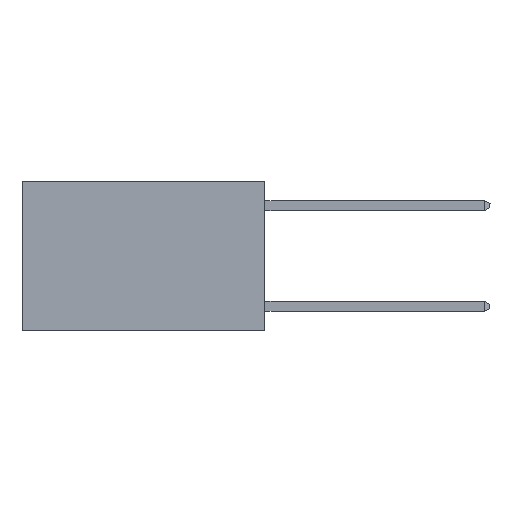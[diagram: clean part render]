
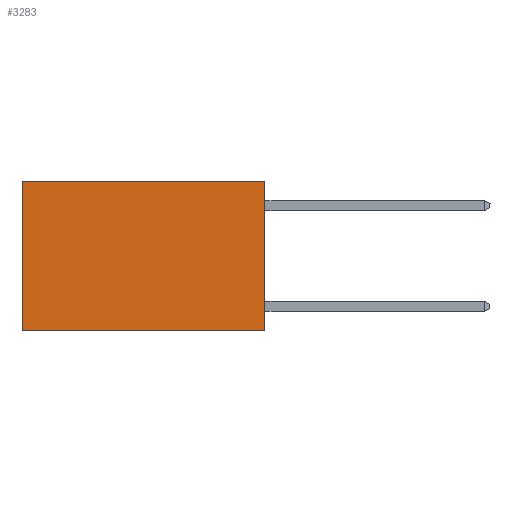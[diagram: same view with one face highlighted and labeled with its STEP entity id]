
A CAD part, left-side view. The second image highlights one B-rep face of the part: STEP entity #3283.
In plain terms, the highlighted planar face has unit normal (-1, 0, 0).
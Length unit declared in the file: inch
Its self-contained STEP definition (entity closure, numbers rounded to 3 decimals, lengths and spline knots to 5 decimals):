
#194 = VECTOR ( 'NONE', #4864, 39.37008 ) ;
#384 = CARTESIAN_POINT ( 'NONE',  ( 0.2625, 0., 0. ) ) ;
#510 = ORIENTED_EDGE ( 'NONE', *, *, #896, .T. ) ;
#896 = EDGE_CURVE ( 'NONE', #1031, #10389, #8297, .T. ) ;
#946 = CARTESIAN_POINT ( 'NONE',  ( 0.2625, 0., -0.37 ) ) ;
#977 = CARTESIAN_POINT ( 'NONE',  ( 0.2625, 0.6, -0.37 ) ) ;
#1031 = VERTEX_POINT ( 'NONE', #7501 ) ;
#1034 = EDGE_CURVE ( 'NONE', #1031, #17882, #9158, .T. ) ;
#3202 = ORIENTED_EDGE ( 'NONE', *, *, #3483, .T. ) ;
#3283 = ADVANCED_FACE ( 'NONE', ( #17440 ), #17118, .F. ) ;
#3401 = VECTOR ( 'NONE', #17740, 39.37008 ) ;
#3483 = EDGE_CURVE ( 'NONE', #10389, #21926, #16109, .T. ) ;
#3780 = CARTESIAN_POINT ( 'NONE',  ( 0.2625, 0., -0.37 ) ) ;
#4864 = DIRECTION ( 'NONE',  ( 0., 1., 0. ) ) ;
#5254 = EDGE_CURVE ( 'NONE', #17882, #21926, #21222, .T. ) ;
#7098 = CARTESIAN_POINT ( 'NONE',  ( 0.2625, 0., 0. ) ) ;
#7501 = CARTESIAN_POINT ( 'NONE',  ( 0.2625, 0., 0. ) ) ;
#7639 = ORIENTED_EDGE ( 'NONE', *, *, #1034, .F. ) ;
#8297 = LINE ( 'NONE', #20116, #194 ) ;
#8539 = VECTOR ( 'NONE', #11180, 39.37008 ) ;
#8653 = DIRECTION ( 'NONE',  ( 0., 0., -1. ) ) ;
#9158 = LINE ( 'NONE', #384, #3401 ) ;
#9390 = CARTESIAN_POINT ( 'NONE',  ( 0.2625, 0.6, 0. ) ) ;
#9549 = ORIENTED_EDGE ( 'NONE', *, *, #5254, .F. ) ;
#10389 = VERTEX_POINT ( 'NONE', #9390 ) ;
#10892 = EDGE_LOOP ( 'NONE', ( #3202, #9549, #7639, #510 ) ) ;
#11180 = DIRECTION ( 'NONE',  ( 0., 1., 0. ) ) ;
#12765 = DIRECTION ( 'NONE',  ( 0., 0., -1. ) ) ;
#14441 = CARTESIAN_POINT ( 'NONE',  ( 0.2625, 0.6, 0. ) ) ;
#14885 = VECTOR ( 'NONE', #12765, 39.37008 ) ;
#16109 = LINE ( 'NONE', #14441, #14885 ) ;
#17118 = PLANE ( 'NONE',  #17722 ) ;
#17331 = DIRECTION ( 'NONE',  ( 1., 0., 0. ) ) ;
#17440 = FACE_OUTER_BOUND ( 'NONE', #10892, .T. ) ;
#17722 = AXIS2_PLACEMENT_3D ( 'NONE', #7098, #17331, #8653 ) ;
#17740 = DIRECTION ( 'NONE',  ( 0., 0., -1. ) ) ;
#17882 = VERTEX_POINT ( 'NONE', #3780 ) ;
#20116 = CARTESIAN_POINT ( 'NONE',  ( 0.2625, 0., 0. ) ) ;
#21222 = LINE ( 'NONE', #946, #8539 ) ;
#21926 = VERTEX_POINT ( 'NONE', #977 ) ;
